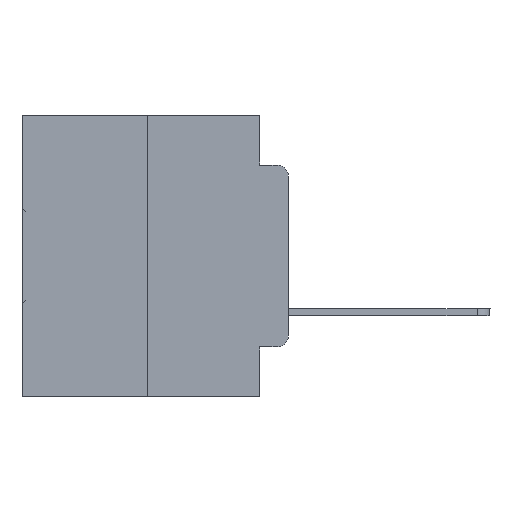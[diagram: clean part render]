
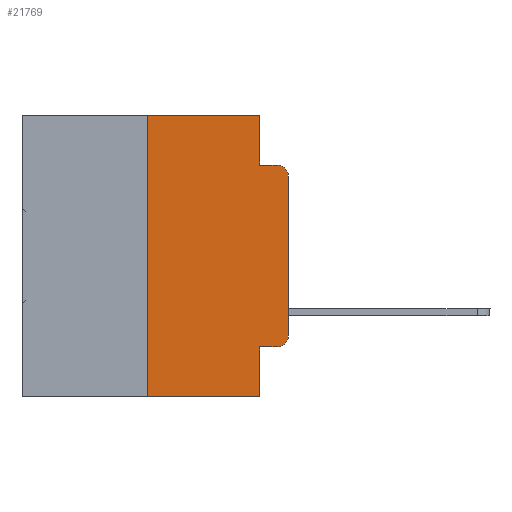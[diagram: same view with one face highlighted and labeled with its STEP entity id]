
A CAD part, left-side view. The second image highlights one B-rep face of the part: STEP entity #21769.
In plain terms, the highlighted planar face has unit normal (-1, 0, 0).
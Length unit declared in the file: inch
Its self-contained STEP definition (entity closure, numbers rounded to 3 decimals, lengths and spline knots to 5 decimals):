
#56 = CARTESIAN_POINT ( 'NONE',  ( 0., 0., 0. ) ) ;
#119 = VERTEX_POINT ( 'NONE', #14532 ) ;
#662 = DIRECTION ( 'NONE',  ( 0., 0., -1. ) ) ;
#1063 = ORIENTED_EDGE ( 'NONE', *, *, #20684, .F. ) ;
#1295 = CARTESIAN_POINT ( 'NONE',  ( 0., 0.051, -0.0885 ) ) ;
#1610 = CARTESIAN_POINT ( 'NONE',  ( 0., 0., -0.3915 ) ) ;
#3011 = LINE ( 'NONE', #15280, #17319 ) ;
#3187 = VERTEX_POINT ( 'NONE', #7325 ) ;
#3509 = CARTESIAN_POINT ( 'NONE',  ( 0., 0., -0.1085 ) ) ;
#4019 = VERTEX_POINT ( 'NONE', #13405 ) ;
#4599 = LINE ( 'NONE', #11887, #9149 ) ;
#5418 = VERTEX_POINT ( 'NONE', #1295 ) ;
#5452 = LINE ( 'NONE', #15301, #9217 ) ;
#5889 = EDGE_CURVE ( 'NONE', #119, #20071, #25440, .T. ) ;
#6337 = ORIENTED_EDGE ( 'NONE', *, *, #5889, .T. ) ;
#6365 = CIRCLE ( 'NONE', #6895, 0.02 ) ;
#6722 = DIRECTION ( 'NONE',  ( 0., -1., 0. ) ) ;
#6740 = DIRECTION ( 'NONE',  ( -1., 0., 0. ) ) ;
#6895 = AXIS2_PLACEMENT_3D ( 'NONE', #19342, #9335, #16278 ) ;
#7325 = CARTESIAN_POINT ( 'NONE',  ( 0., 0.051, -0.5 ) ) ;
#7327 = EDGE_CURVE ( 'NONE', #28394, #5418, #11950, .T. ) ;
#7364 = AXIS2_PLACEMENT_3D ( 'NONE', #16441, #6740, #26792 ) ;
#7855 = DIRECTION ( 'NONE',  ( 0., 0., -1. ) ) ;
#8792 = EDGE_CURVE ( 'NONE', #4019, #28394, #26362, .T. ) ;
#8998 = CARTESIAN_POINT ( 'NONE',  ( 0., 0.473, -0.5 ) ) ;
#9149 = VECTOR ( 'NONE', #29037, 39.37008 ) ;
#9217 = VECTOR ( 'NONE', #18375, 39.37008 ) ;
#9335 = DIRECTION ( 'NONE',  ( -1., 0., 0. ) ) ;
#9821 = LINE ( 'NONE', #26650, #23007 ) ;
#9828 = ORIENTED_EDGE ( 'NONE', *, *, #7327, .F. ) ;
#10158 = VERTEX_POINT ( 'NONE', #26844 ) ;
#10377 = CARTESIAN_POINT ( 'NONE',  ( 0., 0.473, 0. ) ) ;
#10510 = EDGE_CURVE ( 'NONE', #5418, #23636, #9821, .T. ) ;
#11776 = VECTOR ( 'NONE', #22684, 39.37008 ) ;
#11842 = EDGE_CURVE ( 'NONE', #19577, #119, #4599, .T. ) ;
#11887 = CARTESIAN_POINT ( 'NONE',  ( 0., 0.051, -0.4115 ) ) ;
#11936 = ORIENTED_EDGE ( 'NONE', *, *, #31568, .T. ) ;
#11950 = LINE ( 'NONE', #15439, #26557 ) ;
#12854 = CARTESIAN_POINT ( 'NONE',  ( 0., 0.02, -0.0885 ) ) ;
#13405 = CARTESIAN_POINT ( 'NONE',  ( 0., 0.25, 0. ) ) ;
#13505 = LINE ( 'NONE', #8998, #31390 ) ;
#13573 = EDGE_CURVE ( 'NONE', #10158, #3187, #13505, .T. ) ;
#13605 = VECTOR ( 'NONE', #23619, 39.37008 ) ;
#14285 = ORIENTED_EDGE ( 'NONE', *, *, #22436, .T. ) ;
#14532 = CARTESIAN_POINT ( 'NONE',  ( 0., 0.02, -0.4115 ) ) ;
#14598 = VERTEX_POINT ( 'NONE', #3509 ) ;
#14701 = EDGE_CURVE ( 'NONE', #10158, #4019, #5452, .T. ) ;
#14914 = EDGE_LOOP ( 'NONE', ( #14285, #11936, #26022, #9828, #20528, #26290, #15821, #1063, #19208, #6337 ) ) ;
#15280 = CARTESIAN_POINT ( 'NONE',  ( 0., 0.051, 0. ) ) ;
#15301 = CARTESIAN_POINT ( 'NONE',  ( 0., 0.25, 0. ) ) ;
#15439 = CARTESIAN_POINT ( 'NONE',  ( 0., 0.051, 0. ) ) ;
#15821 = ORIENTED_EDGE ( 'NONE', *, *, #13573, .T. ) ;
#16011 = CARTESIAN_POINT ( 'NONE',  ( 0., 0.473, 0. ) ) ;
#16278 = DIRECTION ( 'NONE',  ( 0., 0., -1. ) ) ;
#16441 = CARTESIAN_POINT ( 'NONE',  ( 0., 0.02, -0.3915 ) ) ;
#17319 = VECTOR ( 'NONE', #7855, 39.37008 ) ;
#17869 = CARTESIAN_POINT ( 'NONE',  ( 0., 0.051, -0.4115 ) ) ;
#18276 = DIRECTION ( 'NONE',  ( 1., 0., 0. ) ) ;
#18375 = DIRECTION ( 'NONE',  ( 0., 0., 1. ) ) ;
#19208 = ORIENTED_EDGE ( 'NONE', *, *, #11842, .T. ) ;
#19342 = CARTESIAN_POINT ( 'NONE',  ( 0., 0.02, -0.1085 ) ) ;
#19577 = VERTEX_POINT ( 'NONE', #17869 ) ;
#19657 = DIRECTION ( 'NONE',  ( 0., -1., 0. ) ) ;
#20071 = VERTEX_POINT ( 'NONE', #1610 ) ;
#20528 = ORIENTED_EDGE ( 'NONE', *, *, #8792, .F. ) ;
#20684 = EDGE_CURVE ( 'NONE', #19577, #3187, #3011, .T. ) ;
#20704 = PLANE ( 'NONE',  #23084 ) ;
#21769 = ADVANCED_FACE ( 'NONE', ( #23298 ), #20704, .F. ) ;
#22198 = LINE ( 'NONE', #56, #11776 ) ;
#22436 = EDGE_CURVE ( 'NONE', #20071, #14598, #22198, .T. ) ;
#22684 = DIRECTION ( 'NONE',  ( 0., 0., 1. ) ) ;
#23007 = VECTOR ( 'NONE', #19657, 39.37008 ) ;
#23084 = AXIS2_PLACEMENT_3D ( 'NONE', #10377, #18276, #662 ) ;
#23298 = FACE_OUTER_BOUND ( 'NONE', #14914, .T. ) ;
#23619 = DIRECTION ( 'NONE',  ( 0., -1., 0. ) ) ;
#23636 = VERTEX_POINT ( 'NONE', #12854 ) ;
#25315 = DIRECTION ( 'NONE',  ( 0., 0., -1. ) ) ;
#25440 = CIRCLE ( 'NONE', #7364, 0.02 ) ;
#26022 = ORIENTED_EDGE ( 'NONE', *, *, #10510, .F. ) ;
#26290 = ORIENTED_EDGE ( 'NONE', *, *, #14701, .F. ) ;
#26362 = LINE ( 'NONE', #16011, #13605 ) ;
#26557 = VECTOR ( 'NONE', #25315, 39.37008 ) ;
#26650 = CARTESIAN_POINT ( 'NONE',  ( 0., 0.051, -0.0885 ) ) ;
#26792 = DIRECTION ( 'NONE',  ( 0., 0., -1. ) ) ;
#26844 = CARTESIAN_POINT ( 'NONE',  ( 0., 0.25, -0.5 ) ) ;
#28394 = VERTEX_POINT ( 'NONE', #29922 ) ;
#29037 = DIRECTION ( 'NONE',  ( 0., -1., 0. ) ) ;
#29922 = CARTESIAN_POINT ( 'NONE',  ( 0., 0.051, 0. ) ) ;
#31390 = VECTOR ( 'NONE', #6722, 39.37008 ) ;
#31568 = EDGE_CURVE ( 'NONE', #14598, #23636, #6365, .T. ) ;
